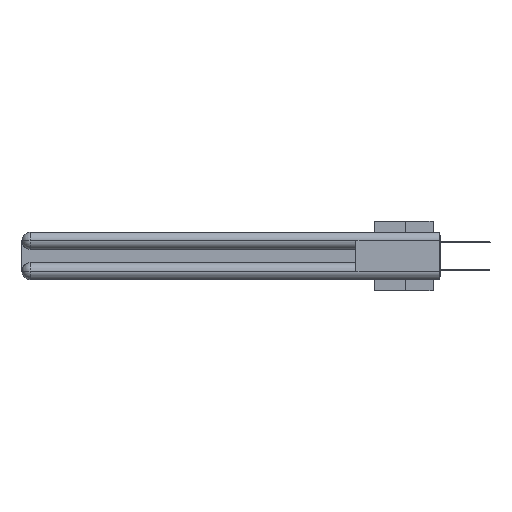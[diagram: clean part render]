
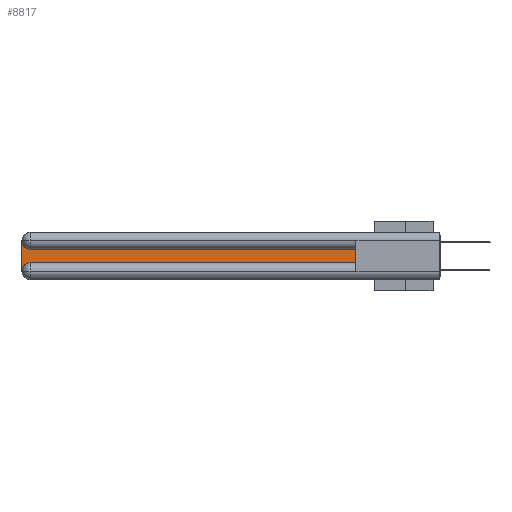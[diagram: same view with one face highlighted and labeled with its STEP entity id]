
A CAD part, left-side view. The second image highlights one B-rep face of the part: STEP entity #8817.
In plain terms, the highlighted planar face has unit normal (-1, 0, 0).
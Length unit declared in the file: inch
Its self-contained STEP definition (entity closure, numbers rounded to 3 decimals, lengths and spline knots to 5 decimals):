
#706 = VERTEX_POINT ( 'NONE', #26919 ) ;
#839 = CARTESIAN_POINT ( 'NONE',  ( 0.075, 3., -0.2175 ) ) ;
#1025 = DIRECTION ( 'NONE',  ( 1., 0., 0. ) ) ;
#1269 = CARTESIAN_POINT ( 'NONE',  ( 0.075, 3., -0.0625 ) ) ;
#1440 = LINE ( 'NONE', #16798, #7538 ) ;
#2245 = EDGE_CURVE ( 'NONE', #22400, #28478, #15380, .T. ) ;
#2363 = ORIENTED_EDGE ( 'NONE', *, *, #19747, .T. ) ;
#3000 = EDGE_LOOP ( 'NONE', ( #9173, #2363, #6892, #14373, #6247, #32586 ) ) ;
#3268 = CARTESIAN_POINT ( 'NONE',  ( 0.075, 2.94, -0.2775 ) ) ;
#5989 = DIRECTION ( 'NONE',  ( 0., 1., 0. ) ) ;
#6247 = ORIENTED_EDGE ( 'NONE', *, *, #20225, .T. ) ;
#6855 = VECTOR ( 'NONE', #28484, 39.37008 ) ;
#6892 = ORIENTED_EDGE ( 'NONE', *, *, #15976, .T. ) ;
#7538 = VECTOR ( 'NONE', #26556, 39.37008 ) ;
#8612 = AXIS2_PLACEMENT_3D ( 'NONE', #3268, #16113, #13113 ) ;
#8817 = ADVANCED_FACE ( 'NONE', ( #15702 ), #10722, .F. ) ;
#9151 = CIRCLE ( 'NONE', #8612, 0.06 ) ;
#9173 = ORIENTED_EDGE ( 'NONE', *, *, #2245, .T. ) ;
#9729 = CARTESIAN_POINT ( 'NONE',  ( 0.075, 2.94, -0.1225 ) ) ;
#10722 = PLANE ( 'NONE',  #31828 ) ;
#10753 = LINE ( 'NONE', #839, #6855 ) ;
#11338 = CARTESIAN_POINT ( 'NONE',  ( 0.075, 0.6, -0.1225 ) ) ;
#12045 = VERTEX_POINT ( 'NONE', #27327 ) ;
#12746 = CARTESIAN_POINT ( 'NONE',  ( 0.075, 3., -0.2775 ) ) ;
#13113 = DIRECTION ( 'NONE',  ( 0., 0., -1. ) ) ;
#13351 = AXIS2_PLACEMENT_3D ( 'NONE', #26634, #1025, #18747 ) ;
#13988 = DIRECTION ( 'NONE',  ( 1., 0., 0. ) ) ;
#14373 = ORIENTED_EDGE ( 'NONE', *, *, #31064, .T. ) ;
#15380 = LINE ( 'NONE', #11338, #29741 ) ;
#15702 = FACE_OUTER_BOUND ( 'NONE', #3000, .T. ) ;
#15914 = VERTEX_POINT ( 'NONE', #12746 ) ;
#15976 = EDGE_CURVE ( 'NONE', #29373, #15914, #10753, .T. ) ;
#16113 = DIRECTION ( 'NONE',  ( 1., 0., 0. ) ) ;
#16798 = CARTESIAN_POINT ( 'NONE',  ( 0.075, 0.6, -0.2175 ) ) ;
#18747 = DIRECTION ( 'NONE',  ( 0., 0., -1. ) ) ;
#19143 = DIRECTION ( 'NONE',  ( 0., 0., -1. ) ) ;
#19747 = EDGE_CURVE ( 'NONE', #28478, #29373, #27806, .T. ) ;
#20006 = DIRECTION ( 'NONE',  ( 0., 0., 1. ) ) ;
#20225 = EDGE_CURVE ( 'NONE', #706, #12045, #1440, .T. ) ;
#22400 = VERTEX_POINT ( 'NONE', #26323 ) ;
#22848 = LINE ( 'NONE', #33066, #27563 ) ;
#23091 = CARTESIAN_POINT ( 'NONE',  ( 0.075, 3., -0.1225 ) ) ;
#24419 = EDGE_CURVE ( 'NONE', #12045, #22400, #22848, .T. ) ;
#26323 = CARTESIAN_POINT ( 'NONE',  ( 0.075, 0.6, -0.1225 ) ) ;
#26556 = DIRECTION ( 'NONE',  ( 0., -1., 0. ) ) ;
#26634 = CARTESIAN_POINT ( 'NONE',  ( 0.075, 2.94, -0.0625 ) ) ;
#26919 = CARTESIAN_POINT ( 'NONE',  ( 0.075, 2.94, -0.2175 ) ) ;
#27327 = CARTESIAN_POINT ( 'NONE',  ( 0.075, 0.6, -0.2175 ) ) ;
#27563 = VECTOR ( 'NONE', #20006, 39.37008 ) ;
#27806 = CIRCLE ( 'NONE', #13351, 0.06 ) ;
#28478 = VERTEX_POINT ( 'NONE', #9729 ) ;
#28484 = DIRECTION ( 'NONE',  ( 0., 0., -1. ) ) ;
#29373 = VERTEX_POINT ( 'NONE', #1269 ) ;
#29741 = VECTOR ( 'NONE', #5989, 39.37008 ) ;
#31064 = EDGE_CURVE ( 'NONE', #15914, #706, #9151, .T. ) ;
#31828 = AXIS2_PLACEMENT_3D ( 'NONE', #23091, #13988, #19143 ) ;
#32586 = ORIENTED_EDGE ( 'NONE', *, *, #24419, .T. ) ;
#33066 = CARTESIAN_POINT ( 'NONE',  ( 0.075, 0.6, -0.2175 ) ) ;
